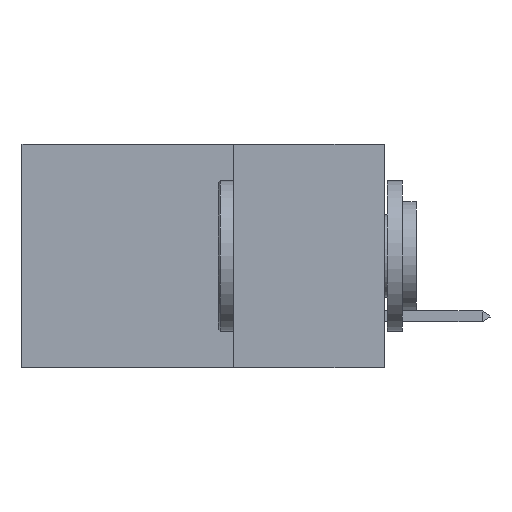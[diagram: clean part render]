
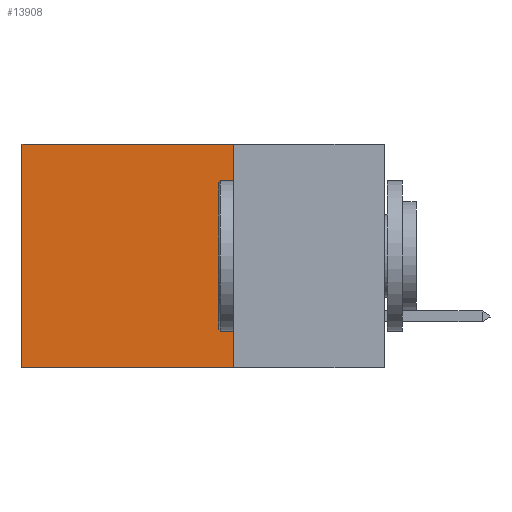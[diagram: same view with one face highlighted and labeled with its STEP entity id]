
A CAD part, left-side view. The second image highlights one B-rep face of the part: STEP entity #13908.
In plain terms, the highlighted planar face has unit normal (-1, 0, 0).
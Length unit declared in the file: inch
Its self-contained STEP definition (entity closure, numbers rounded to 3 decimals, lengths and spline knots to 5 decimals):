
#405 = VECTOR ( 'NONE', #11300, 39.37008 ) ;
#1005 = CARTESIAN_POINT ( 'NONE',  ( 0.2875, 0.25, 0. ) ) ;
#1107 = ORIENTED_EDGE ( 'NONE', *, *, #3131, .F. ) ;
#3131 = EDGE_CURVE ( 'NONE', #31179, #26428, #27364, .T. ) ;
#4362 = CARTESIAN_POINT ( 'NONE',  ( 0.2875, 0.6, 0. ) ) ;
#4943 = ORIENTED_EDGE ( 'NONE', *, *, #17647, .T. ) ;
#5307 = LINE ( 'NONE', #24388, #14472 ) ;
#5701 = DIRECTION ( 'NONE',  ( 0., 0., -1. ) ) ;
#5709 = EDGE_CURVE ( 'NONE', #22390, #31179, #5307, .T. ) ;
#6056 = DIRECTION ( 'NONE',  ( 1., 0., 0. ) ) ;
#6312 = ORIENTED_EDGE ( 'NONE', *, *, #5709, .F. ) ;
#8604 = PLANE ( 'NONE',  #17845 ) ;
#11300 = DIRECTION ( 'NONE',  ( 0., 1., 0. ) ) ;
#11491 = EDGE_CURVE ( 'NONE', #30784, #26428, #12213, .T. ) ;
#12195 = LINE ( 'NONE', #17167, #32442 ) ;
#12213 = LINE ( 'NONE', #17332, #18396 ) ;
#13494 = FACE_OUTER_BOUND ( 'NONE', #30798, .T. ) ;
#13908 = ADVANCED_FACE ( 'NONE', ( #13494 ), #8604, .F. ) ;
#14052 = DIRECTION ( 'NONE',  ( 0., 0., -1. ) ) ;
#14472 = VECTOR ( 'NONE', #5701, 39.37008 ) ;
#17167 = CARTESIAN_POINT ( 'NONE',  ( 0.2875, 0.25, 0. ) ) ;
#17332 = CARTESIAN_POINT ( 'NONE',  ( 0.2875, 0.6, 0. ) ) ;
#17569 = DIRECTION ( 'NONE',  ( 0., 0., -1. ) ) ;
#17647 = EDGE_CURVE ( 'NONE', #22390, #30784, #12195, .T. ) ;
#17845 = AXIS2_PLACEMENT_3D ( 'NONE', #1005, #6056, #14052 ) ;
#18396 = VECTOR ( 'NONE', #17569, 39.37008 ) ;
#21545 = CARTESIAN_POINT ( 'NONE',  ( 0.2875, 0.25, -0.37 ) ) ;
#22390 = VERTEX_POINT ( 'NONE', #30144 ) ;
#22468 = DIRECTION ( 'NONE',  ( 0., 1., 0. ) ) ;
#24388 = CARTESIAN_POINT ( 'NONE',  ( 0.2875, 0.25, 0. ) ) ;
#26428 = VERTEX_POINT ( 'NONE', #29094 ) ;
#27364 = LINE ( 'NONE', #21545, #405 ) ;
#29094 = CARTESIAN_POINT ( 'NONE',  ( 0.2875, 0.6, -0.37 ) ) ;
#29528 = CARTESIAN_POINT ( 'NONE',  ( 0.2875, 0.25, -0.37 ) ) ;
#30144 = CARTESIAN_POINT ( 'NONE',  ( 0.2875, 0.25, 0. ) ) ;
#30784 = VERTEX_POINT ( 'NONE', #4362 ) ;
#30798 = EDGE_LOOP ( 'NONE', ( #32951, #1107, #6312, #4943 ) ) ;
#31179 = VERTEX_POINT ( 'NONE', #29528 ) ;
#32442 = VECTOR ( 'NONE', #22468, 39.37008 ) ;
#32951 = ORIENTED_EDGE ( 'NONE', *, *, #11491, .T. ) ;
